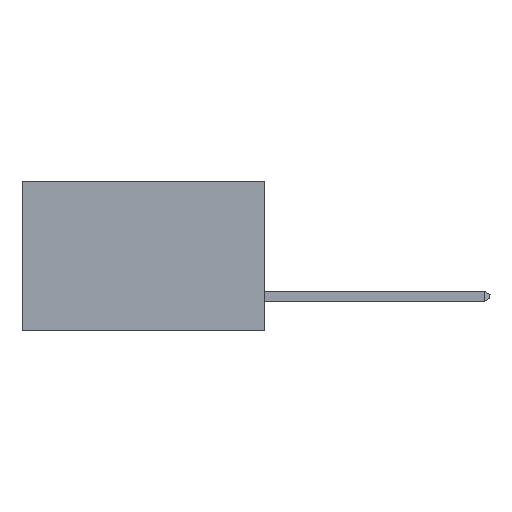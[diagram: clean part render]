
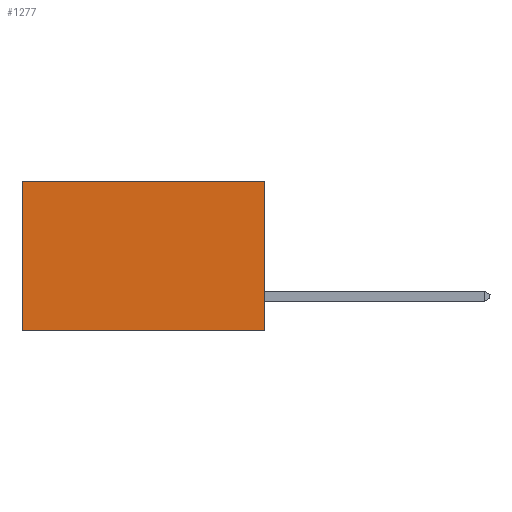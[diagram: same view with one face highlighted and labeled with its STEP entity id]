
A CAD part, left-side view. The second image highlights one B-rep face of the part: STEP entity #1277.
In plain terms, the highlighted planar face has unit normal (-1, 0, 0).
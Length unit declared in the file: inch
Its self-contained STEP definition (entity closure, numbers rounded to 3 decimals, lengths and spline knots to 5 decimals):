
#273 = ORIENTED_EDGE ( 'NONE', *, *, #1059, .T. ) ;
#484 = VECTOR ( 'NONE', #15347, 39.37008 ) ;
#1059 = EDGE_CURVE ( 'NONE', #18669, #6730, #18177, .T. ) ;
#1098 = CARTESIAN_POINT ( 'NONE',  ( 0.2615, 0.6, 0. ) ) ;
#1277 = ADVANCED_FACE ( 'NONE', ( #12685 ), #2476, .F. ) ;
#1311 = CARTESIAN_POINT ( 'NONE',  ( 0.2615, 0.6, -0.37 ) ) ;
#2476 = PLANE ( 'NONE',  #15387 ) ;
#3302 = DIRECTION ( 'NONE',  ( 0., 1., 0. ) ) ;
#3643 = CARTESIAN_POINT ( 'NONE',  ( 0.2615, 0., 0. ) ) ;
#4028 = VECTOR ( 'NONE', #15474, 39.37008 ) ;
#5394 = DIRECTION ( 'NONE',  ( 1., 0., 0. ) ) ;
#5606 = CARTESIAN_POINT ( 'NONE',  ( 0.2615, 0.6, -0.37 ) ) ;
#5664 = ORIENTED_EDGE ( 'NONE', *, *, #13557, .F. ) ;
#6228 = LINE ( 'NONE', #6606, #13815 ) ;
#6444 = VERTEX_POINT ( 'NONE', #1311 ) ;
#6606 = CARTESIAN_POINT ( 'NONE',  ( 0.2615, 0., -0.37 ) ) ;
#6730 = VERTEX_POINT ( 'NONE', #1098 ) ;
#7559 = ORIENTED_EDGE ( 'NONE', *, *, #9686, .F. ) ;
#9686 = EDGE_CURVE ( 'NONE', #18669, #13319, #11138, .T. ) ;
#11138 = LINE ( 'NONE', #17148, #4028 ) ;
#11373 = LINE ( 'NONE', #5606, #15717 ) ;
#12685 = FACE_OUTER_BOUND ( 'NONE', #14798, .T. ) ;
#13070 = DIRECTION ( 'NONE',  ( 0., 0., -1. ) ) ;
#13319 = VERTEX_POINT ( 'NONE', #15800 ) ;
#13557 = EDGE_CURVE ( 'NONE', #13319, #6444, #6228, .T. ) ;
#13815 = VECTOR ( 'NONE', #3302, 39.37008 ) ;
#14798 = EDGE_LOOP ( 'NONE', ( #16579, #5664, #7559, #273 ) ) ;
#14886 = CARTESIAN_POINT ( 'NONE',  ( 0.2615, 0., -0.37 ) ) ;
#15347 = DIRECTION ( 'NONE',  ( 0., 1., 0. ) ) ;
#15387 = AXIS2_PLACEMENT_3D ( 'NONE', #14886, #5394, #15418 ) ;
#15418 = DIRECTION ( 'NONE',  ( 0., 0., -1. ) ) ;
#15474 = DIRECTION ( 'NONE',  ( 0., 0., -1. ) ) ;
#15717 = VECTOR ( 'NONE', #13070, 39.37008 ) ;
#15800 = CARTESIAN_POINT ( 'NONE',  ( 0.2615, 0., -0.37 ) ) ;
#16437 = CARTESIAN_POINT ( 'NONE',  ( 0.2615, 0., 0. ) ) ;
#16579 = ORIENTED_EDGE ( 'NONE', *, *, #17849, .T. ) ;
#17148 = CARTESIAN_POINT ( 'NONE',  ( 0.2615, 0., -0.37 ) ) ;
#17849 = EDGE_CURVE ( 'NONE', #6730, #6444, #11373, .T. ) ;
#18177 = LINE ( 'NONE', #3643, #484 ) ;
#18669 = VERTEX_POINT ( 'NONE', #16437 ) ;
